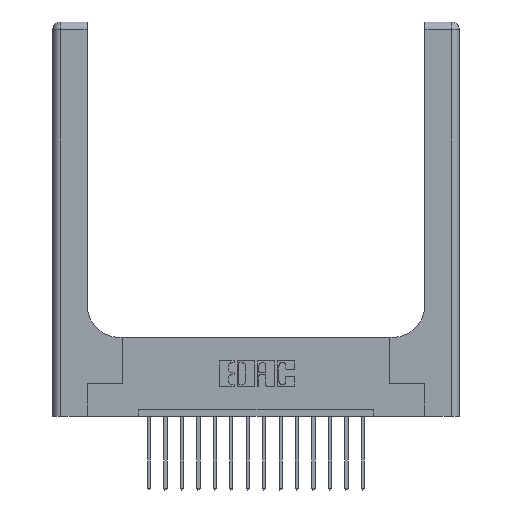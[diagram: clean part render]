
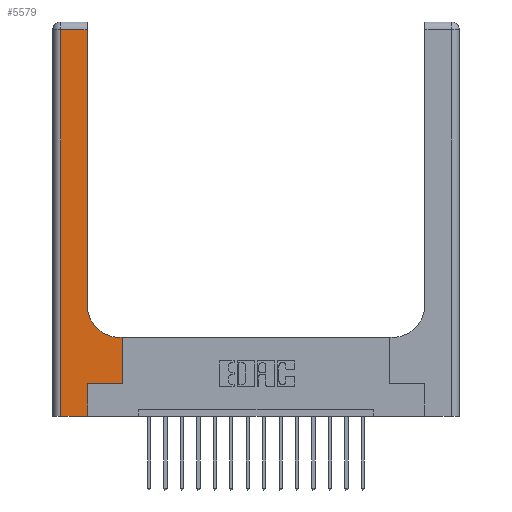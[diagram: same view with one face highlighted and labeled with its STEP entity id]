
A CAD part, top view. The second image highlights one B-rep face of the part: STEP entity #5579.
In plain terms, the highlighted planar face has unit normal (0, 0, 1).
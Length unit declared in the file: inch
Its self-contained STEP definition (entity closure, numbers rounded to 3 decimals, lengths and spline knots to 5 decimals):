
#7 = VECTOR ( 'NONE', #9825, 39.37008 ) ;
#137 = LINE ( 'NONE', #9743, #7 ) ;
#183 = ORIENTED_EDGE ( 'NONE', *, *, #8500, .T. ) ;
#1562 = EDGE_CURVE ( 'NONE', #7154, #14317, #8050, .T. ) ;
#1658 = CARTESIAN_POINT ( 'NONE',  ( 0.265, 0.25, 0.37 ) ) ;
#1799 = CARTESIAN_POINT ( 'NONE',  ( 0.528, 0.25, 0.37 ) ) ;
#1979 = DIRECTION ( 'NONE',  ( -1., 0., 0. ) ) ;
#2167 = ORIENTED_EDGE ( 'NONE', *, *, #17601, .T. ) ;
#2396 = PLANE ( 'NONE',  #3030 ) ;
#2516 = EDGE_CURVE ( 'NONE', #6583, #14522, #4601, .T. ) ;
#2668 = CIRCLE ( 'NONE', #11704, 0.25 ) ;
#2899 = DIRECTION ( 'NONE',  ( 0., 1., 0. ) ) ;
#3030 = AXIS2_PLACEMENT_3D ( 'NONE', #7944, #17937, #12253 ) ;
#3270 = EDGE_CURVE ( 'NONE', #14522, #9932, #4467, .T. ) ;
#3659 = CARTESIAN_POINT ( 'NONE',  ( 0.06, 0., 0.37 ) ) ;
#3662 = LINE ( 'NONE', #6483, #6313 ) ;
#4467 = LINE ( 'NONE', #1799, #10749 ) ;
#4579 = VECTOR ( 'NONE', #1979, 39.37008 ) ;
#4601 = LINE ( 'NONE', #1658, #15302 ) ;
#5102 = CARTESIAN_POINT ( 'NONE',  ( 0., 2.94, 0.37 ) ) ;
#5572 = ORIENTED_EDGE ( 'NONE', *, *, #3270, .T. ) ;
#5579 = ADVANCED_FACE ( 'NONE', ( #13708 ), #2396, .F. ) ;
#5717 = CARTESIAN_POINT ( 'NONE',  ( 0.51, 0.85, 0.37 ) ) ;
#6313 = VECTOR ( 'NONE', #7823, 39.37008 ) ;
#6483 = CARTESIAN_POINT ( 'NONE',  ( 0.265, 0., 0.37 ) ) ;
#6583 = VERTEX_POINT ( 'NONE', #12063 ) ;
#7020 = VERTEX_POINT ( 'NONE', #14686 ) ;
#7154 = VERTEX_POINT ( 'NONE', #3659 ) ;
#7266 = CARTESIAN_POINT ( 'NONE',  ( 0.26, 0.6, 0.37 ) ) ;
#7601 = VECTOR ( 'NONE', #12049, 39.37008 ) ;
#7731 = ORIENTED_EDGE ( 'NONE', *, *, #2516, .T. ) ;
#7809 = LINE ( 'NONE', #5102, #18028 ) ;
#7823 = DIRECTION ( 'NONE',  ( 0., 1., 0. ) ) ;
#7944 = CARTESIAN_POINT ( 'NONE',  ( 0., 3., 0.37 ) ) ;
#8022 = ORIENTED_EDGE ( 'NONE', *, *, #17854, .T. ) ;
#8050 = LINE ( 'NONE', #15283, #10531 ) ;
#8238 = VERTEX_POINT ( 'NONE', #12217 ) ;
#8272 = DIRECTION ( 'NONE',  ( 1., 0., 0. ) ) ;
#8291 = EDGE_CURVE ( 'NONE', #14317, #6583, #3662, .T. ) ;
#8299 = EDGE_LOOP ( 'NONE', ( #2167, #15814, #18019, #15462, #9117, #7731, #5572, #183, #8022 ) ) ;
#8324 = DIRECTION ( 'NONE',  ( 1., 0., 0. ) ) ;
#8351 = CARTESIAN_POINT ( 'NONE',  ( 0.528, 0.25, 0.37 ) ) ;
#8500 = EDGE_CURVE ( 'NONE', #9932, #7020, #13763, .T. ) ;
#9117 = ORIENTED_EDGE ( 'NONE', *, *, #8291, .T. ) ;
#9743 = CARTESIAN_POINT ( 'NONE',  ( 0.06, 3., 0.37 ) ) ;
#9825 = DIRECTION ( 'NONE',  ( 0., -1., 0. ) ) ;
#9879 = DIRECTION ( 'NONE',  ( 1., 0., 0. ) ) ;
#9932 = VERTEX_POINT ( 'NONE', #12108 ) ;
#10415 = CARTESIAN_POINT ( 'NONE',  ( 0.26, 2.94, 0.37 ) ) ;
#10531 = VECTOR ( 'NONE', #8324, 39.37008 ) ;
#10749 = VECTOR ( 'NONE', #2899, 39.37008 ) ;
#10943 = CARTESIAN_POINT ( 'NONE',  ( 0.26, 3., 0.37 ) ) ;
#11175 = VERTEX_POINT ( 'NONE', #11480 ) ;
#11292 = DIRECTION ( 'NONE',  ( 0., 0., -1. ) ) ;
#11480 = CARTESIAN_POINT ( 'NONE',  ( 0.06, 2.94, 0.37 ) ) ;
#11551 = EDGE_CURVE ( 'NONE', #13946, #11175, #7809, .T. ) ;
#11704 = AXIS2_PLACEMENT_3D ( 'NONE', #5717, #11292, #8272 ) ;
#12049 = DIRECTION ( 'NONE',  ( 0., 1., 0. ) ) ;
#12063 = CARTESIAN_POINT ( 'NONE',  ( 0.265, 0.25, 0.37 ) ) ;
#12108 = CARTESIAN_POINT ( 'NONE',  ( 0.528, 0.6, 0.37 ) ) ;
#12217 = CARTESIAN_POINT ( 'NONE',  ( 0.26, 0.85, 0.37 ) ) ;
#12253 = DIRECTION ( 'NONE',  ( -1., 0., 0. ) ) ;
#13708 = FACE_OUTER_BOUND ( 'NONE', #8299, .T. ) ;
#13763 = LINE ( 'NONE', #7266, #4579 ) ;
#13946 = VERTEX_POINT ( 'NONE', #10415 ) ;
#14317 = VERTEX_POINT ( 'NONE', #14683 ) ;
#14522 = VERTEX_POINT ( 'NONE', #8351 ) ;
#14683 = CARTESIAN_POINT ( 'NONE',  ( 0.265, 0., 0.37 ) ) ;
#14686 = CARTESIAN_POINT ( 'NONE',  ( 0.51, 0.6, 0.37 ) ) ;
#15283 = CARTESIAN_POINT ( 'NONE',  ( 0., 0., 0.37 ) ) ;
#15302 = VECTOR ( 'NONE', #9879, 39.37008 ) ;
#15462 = ORIENTED_EDGE ( 'NONE', *, *, #1562, .T. ) ;
#15811 = EDGE_CURVE ( 'NONE', #11175, #7154, #137, .T. ) ;
#15814 = ORIENTED_EDGE ( 'NONE', *, *, #11551, .T. ) ;
#16170 = DIRECTION ( 'NONE',  ( -1., 0., 0. ) ) ;
#16533 = LINE ( 'NONE', #10943, #7601 ) ;
#17601 = EDGE_CURVE ( 'NONE', #8238, #13946, #16533, .T. ) ;
#17854 = EDGE_CURVE ( 'NONE', #7020, #8238, #2668, .T. ) ;
#17937 = DIRECTION ( 'NONE',  ( 0., 0., -1. ) ) ;
#18019 = ORIENTED_EDGE ( 'NONE', *, *, #15811, .T. ) ;
#18028 = VECTOR ( 'NONE', #16170, 39.37008 ) ;
